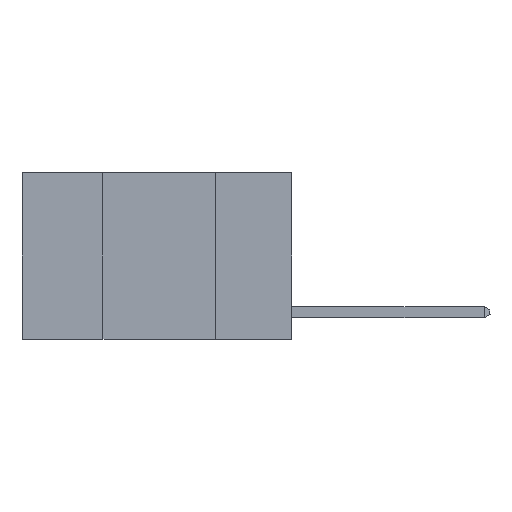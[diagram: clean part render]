
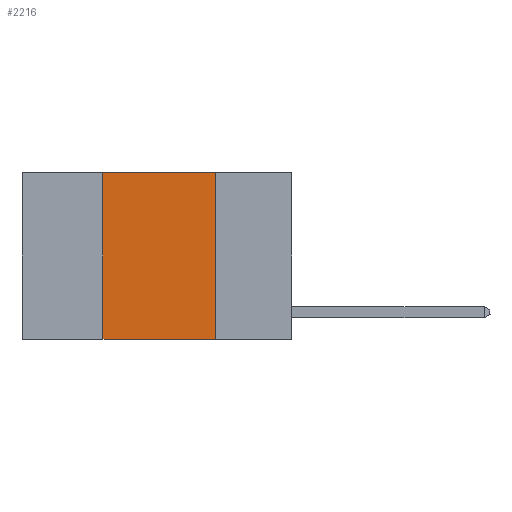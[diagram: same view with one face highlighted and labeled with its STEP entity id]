
A CAD part, left-side view. The second image highlights one B-rep face of the part: STEP entity #2216.
In plain terms, the highlighted planar face has unit normal (-1, 0, 0).
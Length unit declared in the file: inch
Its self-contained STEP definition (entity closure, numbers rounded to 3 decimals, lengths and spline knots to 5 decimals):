
#156 = LINE ( 'NONE', #2233, #4067 ) ;
#293 = PLANE ( 'NONE',  #10520 ) ;
#450 = LINE ( 'NONE', #10618, #3384 ) ;
#539 = CARTESIAN_POINT ( 'NONE',  ( 0., 0.42, 0. ) ) ;
#702 = EDGE_CURVE ( 'NONE', #1266, #6751, #450, .T. ) ;
#810 = EDGE_LOOP ( 'NONE', ( #3753, #6939, #8770, #1753 ) ) ;
#917 = CARTESIAN_POINT ( 'NONE',  ( 0., 0.17, 0. ) ) ;
#1266 = VERTEX_POINT ( 'NONE', #539 ) ;
#1753 = ORIENTED_EDGE ( 'NONE', *, *, #2939, .T. ) ;
#2216 = ADVANCED_FACE ( 'NONE', ( #12891 ), #293, .F. ) ;
#2233 = CARTESIAN_POINT ( 'NONE',  ( 0., 0.42, 0. ) ) ;
#2939 = EDGE_CURVE ( 'NONE', #4321, #8667, #12579, .T. ) ;
#3004 = CARTESIAN_POINT ( 'NONE',  ( 0., 0.42, -0.37 ) ) ;
#3384 = VECTOR ( 'NONE', #4474, 39.37008 ) ;
#3386 = EDGE_CURVE ( 'NONE', #4321, #1266, #156, .T. ) ;
#3753 = ORIENTED_EDGE ( 'NONE', *, *, #5732, .F. ) ;
#4067 = VECTOR ( 'NONE', #4249, 39.37008 ) ;
#4249 = DIRECTION ( 'NONE',  ( 0., 0., 1. ) ) ;
#4321 = VERTEX_POINT ( 'NONE', #3004 ) ;
#4474 = DIRECTION ( 'NONE',  ( 0., -1., 0. ) ) ;
#5399 = DIRECTION ( 'NONE',  ( 0., -1., 0. ) ) ;
#5580 = DIRECTION ( 'NONE',  ( 1., 0., 0. ) ) ;
#5732 = EDGE_CURVE ( 'NONE', #6751, #8667, #6089, .T. ) ;
#6089 = LINE ( 'NONE', #917, #8636 ) ;
#6619 = DIRECTION ( 'NONE',  ( 0., 0., -1. ) ) ;
#6751 = VERTEX_POINT ( 'NONE', #8695 ) ;
#6845 = CARTESIAN_POINT ( 'NONE',  ( 0., 0.17, -0.37 ) ) ;
#6939 = ORIENTED_EDGE ( 'NONE', *, *, #702, .F. ) ;
#7326 = DIRECTION ( 'NONE',  ( 0., 0., -1. ) ) ;
#8636 = VECTOR ( 'NONE', #7326, 39.37008 ) ;
#8667 = VERTEX_POINT ( 'NONE', #6845 ) ;
#8695 = CARTESIAN_POINT ( 'NONE',  ( 0., 0.17, 0. ) ) ;
#8770 = ORIENTED_EDGE ( 'NONE', *, *, #3386, .F. ) ;
#10484 = CARTESIAN_POINT ( 'NONE',  ( 0., 0.6, -0.37 ) ) ;
#10520 = AXIS2_PLACEMENT_3D ( 'NONE', #11565, #5580, #6619 ) ;
#10618 = CARTESIAN_POINT ( 'NONE',  ( 0., 0.6, 0. ) ) ;
#10758 = VECTOR ( 'NONE', #5399, 39.37008 ) ;
#11565 = CARTESIAN_POINT ( 'NONE',  ( 0., 0.6, 0. ) ) ;
#12579 = LINE ( 'NONE', #10484, #10758 ) ;
#12891 = FACE_OUTER_BOUND ( 'NONE', #810, .T. ) ;
